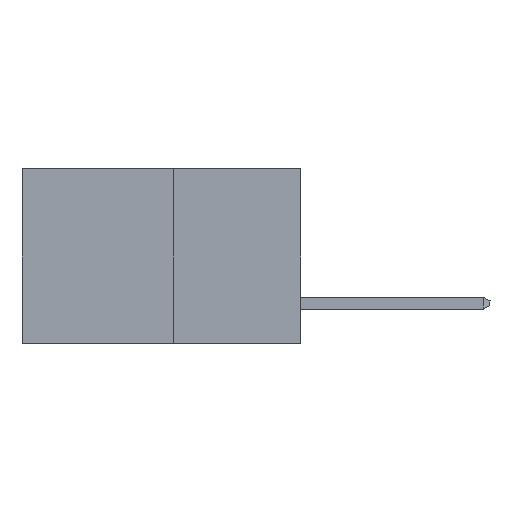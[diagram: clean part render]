
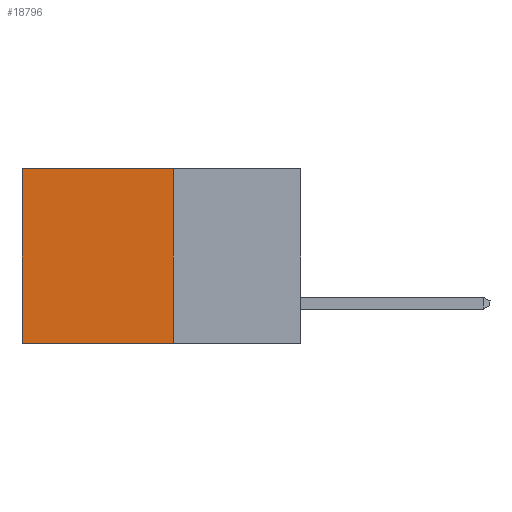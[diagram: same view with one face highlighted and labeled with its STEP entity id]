
A CAD part, left-side view. The second image highlights one B-rep face of the part: STEP entity #18796.
In plain terms, the highlighted planar face has unit normal (-1, 0, 0).
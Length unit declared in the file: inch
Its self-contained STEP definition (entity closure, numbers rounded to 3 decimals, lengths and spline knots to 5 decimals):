
#494 = CARTESIAN_POINT ( 'NONE',  ( 0.277, 0.27, 0. ) ) ;
#1095 = CARTESIAN_POINT ( 'NONE',  ( 0.277, 0.27, -0.37 ) ) ;
#3572 = PLANE ( 'NONE',  #17232 ) ;
#3822 = VERTEX_POINT ( 'NONE', #20791 ) ;
#4283 = ORIENTED_EDGE ( 'NONE', *, *, #8639, .T. ) ;
#4308 = ORIENTED_EDGE ( 'NONE', *, *, #13608, .F. ) ;
#4341 = LINE ( 'NONE', #19620, #13692 ) ;
#5432 = ORIENTED_EDGE ( 'NONE', *, *, #10287, .F. ) ;
#5478 = ORIENTED_EDGE ( 'NONE', *, *, #8825, .T. ) ;
#5535 = DIRECTION ( 'NONE',  ( 1., 0., 0. ) ) ;
#7033 = LINE ( 'NONE', #22365, #21243 ) ;
#8639 = EDGE_CURVE ( 'NONE', #20097, #3822, #12856, .T. ) ;
#8825 = EDGE_CURVE ( 'NONE', #20983, #20097, #4341, .T. ) ;
#9343 = DIRECTION ( 'NONE',  ( 0., 1., 0. ) ) ;
#9995 = EDGE_LOOP ( 'NONE', ( #4283, #4308, #5432, #5478 ) ) ;
#10287 = EDGE_CURVE ( 'NONE', #20983, #12120, #20573, .T. ) ;
#10424 = DIRECTION ( 'NONE',  ( 0., 1., 0. ) ) ;
#11120 = CARTESIAN_POINT ( 'NONE',  ( 0.277, 0.27, -0.37 ) ) ;
#12120 = VERTEX_POINT ( 'NONE', #1095 ) ;
#12856 = LINE ( 'NONE', #15158, #17136 ) ;
#13533 = FACE_OUTER_BOUND ( 'NONE', #9995, .T. ) ;
#13608 = EDGE_CURVE ( 'NONE', #12120, #3822, #7033, .T. ) ;
#13692 = VECTOR ( 'NONE', #10424, 39.37008 ) ;
#15158 = CARTESIAN_POINT ( 'NONE',  ( 0.277, 0.59, -0.37 ) ) ;
#15630 = VECTOR ( 'NONE', #18354, 39.37008 ) ;
#16477 = CARTESIAN_POINT ( 'NONE',  ( 0.277, 0.27, -0.37 ) ) ;
#17136 = VECTOR ( 'NONE', #22645, 39.37008 ) ;
#17232 = AXIS2_PLACEMENT_3D ( 'NONE', #11120, #5535, #18506 ) ;
#18354 = DIRECTION ( 'NONE',  ( 0., 0., -1. ) ) ;
#18506 = DIRECTION ( 'NONE',  ( 0., 0., -1. ) ) ;
#18796 = ADVANCED_FACE ( 'NONE', ( #13533 ), #3572, .F. ) ;
#19620 = CARTESIAN_POINT ( 'NONE',  ( 0.277, 0.27, 0. ) ) ;
#20097 = VERTEX_POINT ( 'NONE', #20582 ) ;
#20573 = LINE ( 'NONE', #16477, #15630 ) ;
#20582 = CARTESIAN_POINT ( 'NONE',  ( 0.277, 0.59, 0. ) ) ;
#20791 = CARTESIAN_POINT ( 'NONE',  ( 0.277, 0.59, -0.37 ) ) ;
#20983 = VERTEX_POINT ( 'NONE', #494 ) ;
#21243 = VECTOR ( 'NONE', #9343, 39.37008 ) ;
#22365 = CARTESIAN_POINT ( 'NONE',  ( 0.277, 0.27, -0.37 ) ) ;
#22645 = DIRECTION ( 'NONE',  ( 0., 0., -1. ) ) ;
